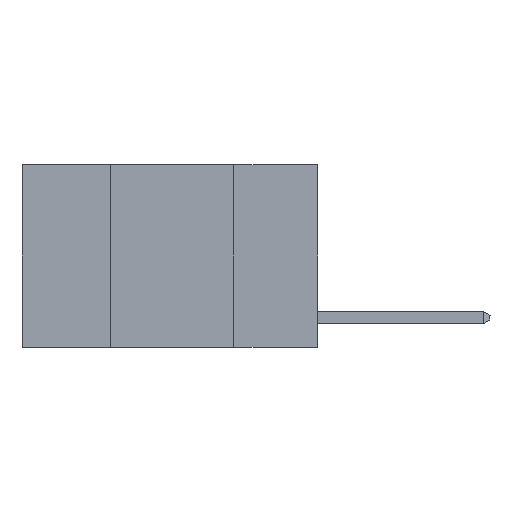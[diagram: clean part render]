
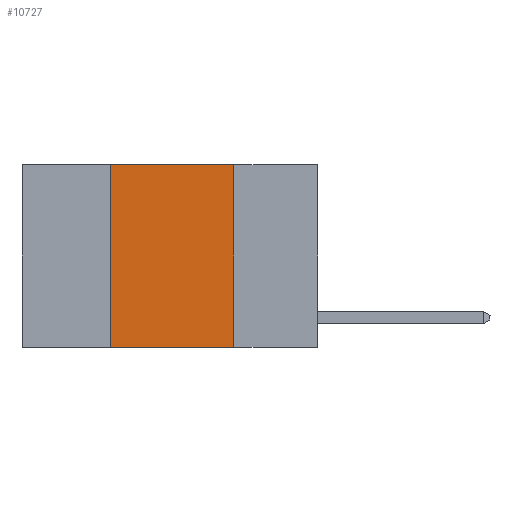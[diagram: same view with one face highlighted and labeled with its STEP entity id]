
A CAD part, left-side view. The second image highlights one B-rep face of the part: STEP entity #10727.
In plain terms, the highlighted planar face has unit normal (-1, 0, 0).
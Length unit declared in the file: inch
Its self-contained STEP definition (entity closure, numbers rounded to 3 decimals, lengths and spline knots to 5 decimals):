
#1087 = CARTESIAN_POINT ( 'NONE',  ( 0., 0.17, -0.37 ) ) ;
#1150 = ORIENTED_EDGE ( 'NONE', *, *, #15656, .F. ) ;
#1233 = EDGE_LOOP ( 'NONE', ( #1150, #2311, #9869, #14188 ) ) ;
#1419 = VERTEX_POINT ( 'NONE', #1087 ) ;
#1532 = LINE ( 'NONE', #2333, #2829 ) ;
#1662 = PLANE ( 'NONE',  #6961 ) ;
#1725 = DIRECTION ( 'NONE',  ( 1., 0., 0. ) ) ;
#1983 = VERTEX_POINT ( 'NONE', #10376 ) ;
#2311 = ORIENTED_EDGE ( 'NONE', *, *, #12616, .F. ) ;
#2333 = CARTESIAN_POINT ( 'NONE',  ( 0., 0.42, 0. ) ) ;
#2829 = VECTOR ( 'NONE', #15753, 39.37008 ) ;
#3168 = CARTESIAN_POINT ( 'NONE',  ( 0., 0.6, 0. ) ) ;
#3295 = VECTOR ( 'NONE', #13273, 39.37008 ) ;
#3761 = CARTESIAN_POINT ( 'NONE',  ( 0., 0.6, -0.37 ) ) ;
#3894 = EDGE_CURVE ( 'NONE', #7143, #1419, #14824, .T. ) ;
#4988 = VECTOR ( 'NONE', #5847, 39.37008 ) ;
#5847 = DIRECTION ( 'NONE',  ( 0., -1., 0. ) ) ;
#6961 = AXIS2_PLACEMENT_3D ( 'NONE', #3168, #1725, #11095 ) ;
#7101 = FACE_OUTER_BOUND ( 'NONE', #1233, .T. ) ;
#7143 = VERTEX_POINT ( 'NONE', #9486 ) ;
#9486 = CARTESIAN_POINT ( 'NONE',  ( 0., 0.42, -0.37 ) ) ;
#9724 = DIRECTION ( 'NONE',  ( 0., 0., -1. ) ) ;
#9869 = ORIENTED_EDGE ( 'NONE', *, *, #17338, .F. ) ;
#10376 = CARTESIAN_POINT ( 'NONE',  ( 0., 0.17, 0. ) ) ;
#10727 = ADVANCED_FACE ( 'NONE', ( #7101 ), #1662, .F. ) ;
#10836 = VERTEX_POINT ( 'NONE', #16708 ) ;
#11095 = DIRECTION ( 'NONE',  ( 0., 0., -1. ) ) ;
#11268 = CARTESIAN_POINT ( 'NONE',  ( 0., 0.6, 0. ) ) ;
#11457 = LINE ( 'NONE', #12390, #16746 ) ;
#12390 = CARTESIAN_POINT ( 'NONE',  ( 0., 0.17, 0. ) ) ;
#12616 = EDGE_CURVE ( 'NONE', #10836, #1983, #15647, .T. ) ;
#13273 = DIRECTION ( 'NONE',  ( 0., -1., 0. ) ) ;
#14188 = ORIENTED_EDGE ( 'NONE', *, *, #3894, .T. ) ;
#14824 = LINE ( 'NONE', #3761, #3295 ) ;
#15647 = LINE ( 'NONE', #11268, #4988 ) ;
#15656 = EDGE_CURVE ( 'NONE', #1983, #1419, #11457, .T. ) ;
#15753 = DIRECTION ( 'NONE',  ( 0., 0., 1. ) ) ;
#16708 = CARTESIAN_POINT ( 'NONE',  ( 0., 0.42, 0. ) ) ;
#16746 = VECTOR ( 'NONE', #9724, 39.37008 ) ;
#17338 = EDGE_CURVE ( 'NONE', #7143, #10836, #1532, .T. ) ;
